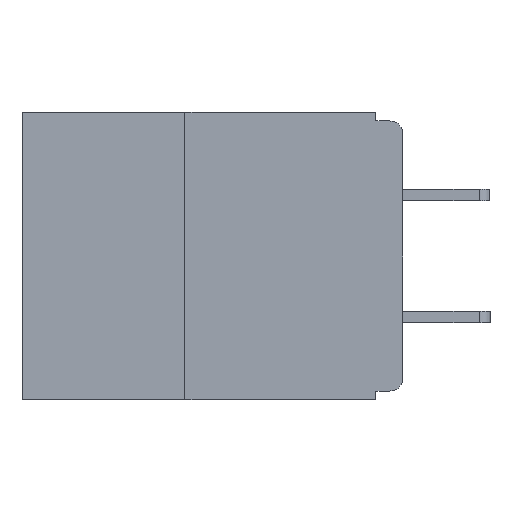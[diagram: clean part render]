
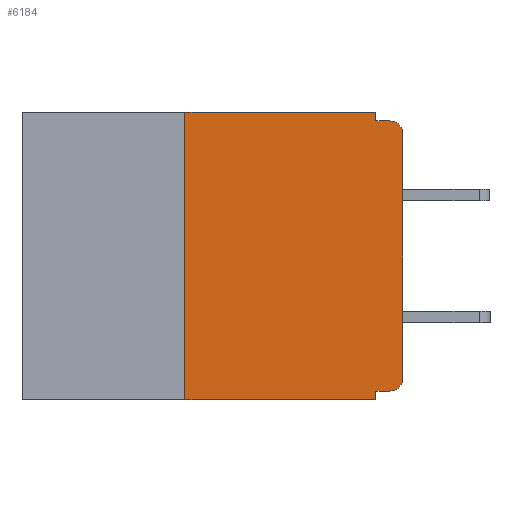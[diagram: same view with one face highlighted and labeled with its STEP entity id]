
A CAD part, left-side view. The second image highlights one B-rep face of the part: STEP entity #6184.
In plain terms, the highlighted planar face has unit normal (-1, 0, 0).
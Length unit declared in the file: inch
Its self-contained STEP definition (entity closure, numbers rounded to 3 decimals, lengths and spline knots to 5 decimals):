
#815 = DIRECTION ( 'NONE',  ( 0., -1., 0. ) ) ;
#1036 = CARTESIAN_POINT ( 'NONE',  ( 0., 0., -0.01 ) ) ;
#1046 = CARTESIAN_POINT ( 'NONE',  ( 0., 0.031, 0. ) ) ;
#1273 = VERTEX_POINT ( 'NONE', #2011 ) ;
#1393 = VERTEX_POINT ( 'NONE', #1737 ) ;
#1641 = EDGE_CURVE ( 'NONE', #11782, #11723, #6306, .T. ) ;
#1715 = CARTESIAN_POINT ( 'NONE',  ( 0., 0.031, 0. ) ) ;
#1717 = EDGE_CURVE ( 'NONE', #1273, #4273, #6236, .T. ) ;
#1737 = CARTESIAN_POINT ( 'NONE',  ( 0., 0.015, -0.01 ) ) ;
#1792 = EDGE_CURVE ( 'NONE', #3623, #7458, #5910, .T. ) ;
#1855 = CARTESIAN_POINT ( 'NONE',  ( 0., 0.437, -0.33 ) ) ;
#1919 = DIRECTION ( 'NONE',  ( 0., -1., 0. ) ) ;
#1980 = FACE_OUTER_BOUND ( 'NONE', #12203, .T. ) ;
#2008 = VECTOR ( 'NONE', #1919, 39.37008 ) ;
#2011 = CARTESIAN_POINT ( 'NONE',  ( 0., 0.25, -0.33 ) ) ;
#2135 = DIRECTION ( 'NONE',  ( 0., 1., 0. ) ) ;
#2204 = LINE ( 'NONE', #1855, #2008 ) ;
#2298 = AXIS2_PLACEMENT_3D ( 'NONE', #6119, #6102, #6015 ) ;
#2305 = CARTESIAN_POINT ( 'NONE',  ( 0., 0., -0.32 ) ) ;
#2564 = CARTESIAN_POINT ( 'NONE',  ( 0., 0.031, -0.32 ) ) ;
#2724 = CARTESIAN_POINT ( 'NONE',  ( 0., 0.25, -0.33 ) ) ;
#2827 = DIRECTION ( 'NONE',  ( 0., 0., 1. ) ) ;
#3016 = VECTOR ( 'NONE', #815, 39.37008 ) ;
#3214 = LINE ( 'NONE', #1036, #3016 ) ;
#3623 = VERTEX_POINT ( 'NONE', #1715 ) ;
#3733 = VECTOR ( 'NONE', #2135, 39.37008 ) ;
#3842 = VECTOR ( 'NONE', #5310, 39.37008 ) ;
#4043 = CIRCLE ( 'NONE', #2298, 0.015 ) ;
#4208 = LINE ( 'NONE', #5284, #3842 ) ;
#4273 = VERTEX_POINT ( 'NONE', #4438 ) ;
#4438 = CARTESIAN_POINT ( 'NONE',  ( 0., 0.25, 0. ) ) ;
#4574 = VECTOR ( 'NONE', #7822, 39.37008 ) ;
#4598 = LINE ( 'NONE', #8275, #4574 ) ;
#4812 = CARTESIAN_POINT ( 'NONE',  ( 0., 0.031, -0.33 ) ) ;
#4977 = CIRCLE ( 'NONE', #7623, 0.015 ) ;
#5033 = AXIS2_PLACEMENT_3D ( 'NONE', #7787, #7638, #7624 ) ;
#5117 = CARTESIAN_POINT ( 'NONE',  ( 0., 0.031, -0.01 ) ) ;
#5284 = CARTESIAN_POINT ( 'NONE',  ( 0., 0.031, -0.33 ) ) ;
#5310 = DIRECTION ( 'NONE',  ( 0., 0., -1. ) ) ;
#5767 = EDGE_CURVE ( 'NONE', #7562, #10561, #4208, .T. ) ;
#5870 = VECTOR ( 'NONE', #8856, 39.37008 ) ;
#5910 = LINE ( 'NONE', #1046, #5870 ) ;
#6015 = DIRECTION ( 'NONE',  ( 0., 0., -1. ) ) ;
#6102 = DIRECTION ( 'NONE',  ( -1., 0., 0. ) ) ;
#6119 = CARTESIAN_POINT ( 'NONE',  ( 0., 0.015, -0.305 ) ) ;
#6137 = VECTOR ( 'NONE', #2827, 39.37008 ) ;
#6151 = LINE ( 'NONE', #2305, #3733 ) ;
#6184 = ADVANCED_FACE ( 'NONE', ( #1980 ), #8040, .F. ) ;
#6236 = LINE ( 'NONE', #2724, #6137 ) ;
#6294 = VECTOR ( 'NONE', #9371, 39.37008 ) ;
#6306 = LINE ( 'NONE', #7006, #6294 ) ;
#6454 = ORIENTED_EDGE ( 'NONE', *, *, #1641, .T. ) ;
#6743 = ORIENTED_EDGE ( 'NONE', *, *, #8705, .T. ) ;
#6927 = ORIENTED_EDGE ( 'NONE', *, *, #10914, .F. ) ;
#7006 = CARTESIAN_POINT ( 'NONE',  ( 0., 0., 0. ) ) ;
#7159 = DIRECTION ( 'NONE',  ( 0., 0., -1. ) ) ;
#7186 = DIRECTION ( 'NONE',  ( -1., 0., 0. ) ) ;
#7195 = CARTESIAN_POINT ( 'NONE',  ( 0., 0.015, -0.025 ) ) ;
#7458 = VERTEX_POINT ( 'NONE', #5117 ) ;
#7562 = VERTEX_POINT ( 'NONE', #2564 ) ;
#7623 = AXIS2_PLACEMENT_3D ( 'NONE', #7195, #7186, #7159 ) ;
#7624 = DIRECTION ( 'NONE',  ( 0., 0., -1. ) ) ;
#7638 = DIRECTION ( 'NONE',  ( 1., 0., 0. ) ) ;
#7648 = ORIENTED_EDGE ( 'NONE', *, *, #1792, .F. ) ;
#7669 = ORIENTED_EDGE ( 'NONE', *, *, #12002, .F. ) ;
#7709 = ORIENTED_EDGE ( 'NONE', *, *, #1717, .F. ) ;
#7787 = CARTESIAN_POINT ( 'NONE',  ( 0., 0.437, 0. ) ) ;
#7792 = ORIENTED_EDGE ( 'NONE', *, *, #12440, .T. ) ;
#7805 = ORIENTED_EDGE ( 'NONE', *, *, #5767, .F. ) ;
#7822 = DIRECTION ( 'NONE',  ( 0., -1., 0. ) ) ;
#7879 = ORIENTED_EDGE ( 'NONE', *, *, #9360, .F. ) ;
#7900 = ORIENTED_EDGE ( 'NONE', *, *, #12128, .T. ) ;
#8040 = PLANE ( 'NONE',  #5033 ) ;
#8275 = CARTESIAN_POINT ( 'NONE',  ( 0., 0.437, 0. ) ) ;
#8630 = VERTEX_POINT ( 'NONE', #10266 ) ;
#8705 = EDGE_CURVE ( 'NONE', #11723, #1393, #4977, .T. ) ;
#8856 = DIRECTION ( 'NONE',  ( 0., 0., -1. ) ) ;
#9360 = EDGE_CURVE ( 'NONE', #8630, #7562, #6151, .T. ) ;
#9371 = DIRECTION ( 'NONE',  ( 0., 0., 1. ) ) ;
#10266 = CARTESIAN_POINT ( 'NONE',  ( 0., 0.015, -0.32 ) ) ;
#10561 = VERTEX_POINT ( 'NONE', #4812 ) ;
#10914 = EDGE_CURVE ( 'NONE', #7458, #1393, #3214, .T. ) ;
#11723 = VERTEX_POINT ( 'NONE', #13218 ) ;
#11782 = VERTEX_POINT ( 'NONE', #12077 ) ;
#12002 = EDGE_CURVE ( 'NONE', #4273, #3623, #4598, .T. ) ;
#12077 = CARTESIAN_POINT ( 'NONE',  ( 0., 0., -0.305 ) ) ;
#12128 = EDGE_CURVE ( 'NONE', #8630, #11782, #4043, .T. ) ;
#12203 = EDGE_LOOP ( 'NONE', ( #6454, #6743, #6927, #7648, #7669, #7709, #7792, #7805, #7879, #7900 ) ) ;
#12440 = EDGE_CURVE ( 'NONE', #1273, #10561, #2204, .T. ) ;
#13218 = CARTESIAN_POINT ( 'NONE',  ( 0., 0., -0.025 ) ) ;
